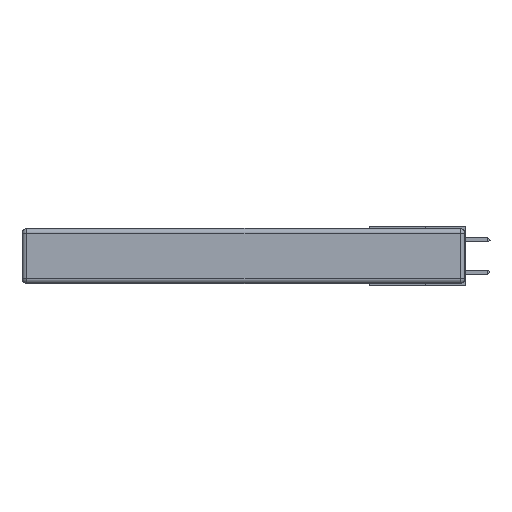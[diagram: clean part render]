
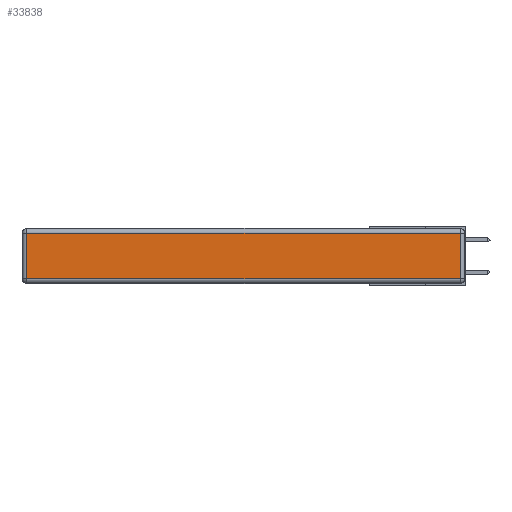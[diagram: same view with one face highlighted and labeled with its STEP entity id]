
A CAD part, left-side view. The second image highlights one B-rep face of the part: STEP entity #33838.
In plain terms, the highlighted planar face has unit normal (-1, 0, 0).
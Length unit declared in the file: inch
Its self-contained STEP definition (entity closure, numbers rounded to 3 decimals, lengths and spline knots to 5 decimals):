
#944 = VECTOR ( 'NONE', #29318, 39.37008 ) ;
#1304 = ORIENTED_EDGE ( 'NONE', *, *, #8710, .T. ) ;
#1367 = LINE ( 'NONE', #31440, #28882 ) ;
#1530 = VERTEX_POINT ( 'NONE', #11699 ) ;
#2195 = CARTESIAN_POINT ( 'NONE',  ( 0., 0., -0.313 ) ) ;
#2382 = EDGE_CURVE ( 'NONE', #20168, #20426, #26555, .T. ) ;
#3689 = ORIENTED_EDGE ( 'NONE', *, *, #7709, .T. ) ;
#4401 = CARTESIAN_POINT ( 'NONE',  ( 0., 2.72, -0.313 ) ) ;
#4905 = ORIENTED_EDGE ( 'NONE', *, *, #2382, .T. ) ;
#5261 = DIRECTION ( 'NONE',  ( 0., 1., 0. ) ) ;
#6625 = DIRECTION ( 'NONE',  ( 0., 0., -1. ) ) ;
#7709 = EDGE_CURVE ( 'NONE', #27901, #1530, #1367, .T. ) ;
#8710 = EDGE_CURVE ( 'NONE', #20426, #27901, #17782, .T. ) ;
#11266 = DIRECTION ( 'NONE',  ( -1., 0., 0. ) ) ;
#11699 = CARTESIAN_POINT ( 'NONE',  ( 0., 2.72, -0.03 ) ) ;
#15584 = AXIS2_PLACEMENT_3D ( 'NONE', #24335, #11266, #24448 ) ;
#16114 = CARTESIAN_POINT ( 'NONE',  ( 0., 0.03, -0.343 ) ) ;
#17782 = LINE ( 'NONE', #16114, #944 ) ;
#19546 = VECTOR ( 'NONE', #33434, 39.37008 ) ;
#20168 = VERTEX_POINT ( 'NONE', #4401 ) ;
#20426 = VERTEX_POINT ( 'NONE', #26237 ) ;
#22576 = VECTOR ( 'NONE', #6625, 39.37008 ) ;
#22969 = LINE ( 'NONE', #30183, #22576 ) ;
#23809 = EDGE_CURVE ( 'NONE', #1530, #20168, #22969, .T. ) ;
#24335 = CARTESIAN_POINT ( 'NONE',  ( 0., 0., -0.343 ) ) ;
#24448 = DIRECTION ( 'NONE',  ( 0., 0., 1. ) ) ;
#24554 = PLANE ( 'NONE',  #15584 ) ;
#26089 = EDGE_LOOP ( 'NONE', ( #4905, #1304, #3689, #32231 ) ) ;
#26237 = CARTESIAN_POINT ( 'NONE',  ( 0., 0.03, -0.313 ) ) ;
#26411 = FACE_OUTER_BOUND ( 'NONE', #26089, .T. ) ;
#26555 = LINE ( 'NONE', #2195, #19546 ) ;
#27901 = VERTEX_POINT ( 'NONE', #33698 ) ;
#28882 = VECTOR ( 'NONE', #5261, 39.37008 ) ;
#29318 = DIRECTION ( 'NONE',  ( 0., 0., 1. ) ) ;
#30183 = CARTESIAN_POINT ( 'NONE',  ( 0., 2.72, -0.343 ) ) ;
#31440 = CARTESIAN_POINT ( 'NONE',  ( 0., 2.75, -0.03 ) ) ;
#32231 = ORIENTED_EDGE ( 'NONE', *, *, #23809, .T. ) ;
#33434 = DIRECTION ( 'NONE',  ( 0., -1., 0. ) ) ;
#33698 = CARTESIAN_POINT ( 'NONE',  ( 0., 0.03, -0.03 ) ) ;
#33838 = ADVANCED_FACE ( 'NONE', ( #26411 ), #24554, .T. ) ;
